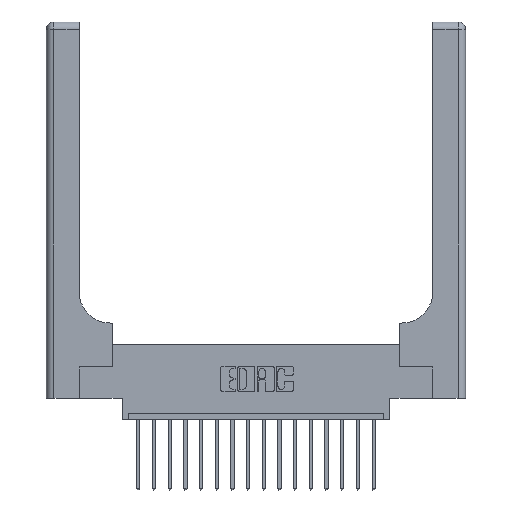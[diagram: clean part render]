
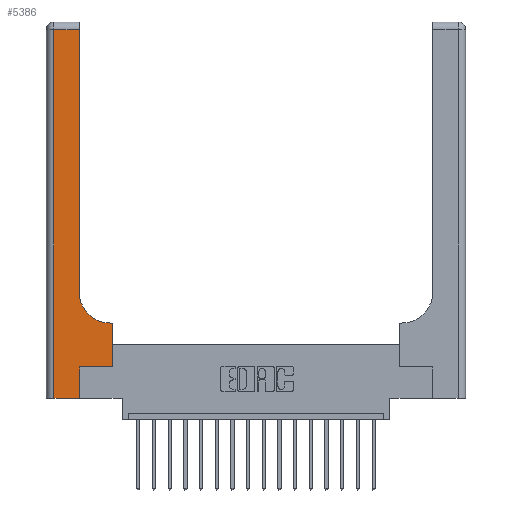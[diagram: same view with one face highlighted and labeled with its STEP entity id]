
A CAD part, top view. The second image highlights one B-rep face of the part: STEP entity #5386.
In plain terms, the highlighted planar face has unit normal (0, 0, 1).
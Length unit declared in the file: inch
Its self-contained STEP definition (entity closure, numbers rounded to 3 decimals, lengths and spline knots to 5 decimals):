
#7 = CARTESIAN_POINT ( 'NONE',  ( 0.51, 0.6, 0.37 ) ) ;
#153 = EDGE_CURVE ( 'NONE', #842, #13573, #8564, .T. ) ;
#242 = ORIENTED_EDGE ( 'NONE', *, *, #1094, .T. ) ;
#585 = EDGE_LOOP ( 'NONE', ( #3375, #5539, #4293, #13679, #2827, #242, #11772, #3308, #14104 ) ) ;
#842 = VERTEX_POINT ( 'NONE', #1672 ) ;
#946 = LINE ( 'NONE', #2567, #9885 ) ;
#1094 = EDGE_CURVE ( 'NONE', #7335, #13065, #18753, .T. ) ;
#1672 = CARTESIAN_POINT ( 'NONE',  ( 0.26, 2.94, 0.37 ) ) ;
#1750 = CARTESIAN_POINT ( 'NONE',  ( 0.528, 0.25, 0.37 ) ) ;
#2262 = LINE ( 'NONE', #8172, #13637 ) ;
#2374 = CARTESIAN_POINT ( 'NONE',  ( 0.265, 0., 0.37 ) ) ;
#2377 = DIRECTION ( 'NONE',  ( -1., 0., 0. ) ) ;
#2567 = CARTESIAN_POINT ( 'NONE',  ( 0.265, 0., 0.37 ) ) ;
#2792 = EDGE_CURVE ( 'NONE', #10053, #8790, #9748, .T. ) ;
#2827 = ORIENTED_EDGE ( 'NONE', *, *, #16114, .T. ) ;
#2954 = FACE_OUTER_BOUND ( 'NONE', #585, .T. ) ;
#3308 = ORIENTED_EDGE ( 'NONE', *, *, #16003, .T. ) ;
#3353 = VECTOR ( 'NONE', #17284, 39.37008 ) ;
#3375 = ORIENTED_EDGE ( 'NONE', *, *, #8252, .T. ) ;
#3729 = VERTEX_POINT ( 'NONE', #7 ) ;
#4293 = ORIENTED_EDGE ( 'NONE', *, *, #9003, .T. ) ;
#4323 = LINE ( 'NONE', #7350, #4621 ) ;
#4621 = VECTOR ( 'NONE', #8796, 39.37008 ) ;
#5386 = ADVANCED_FACE ( 'NONE', ( #2954 ), #8999, .F. ) ;
#5539 = ORIENTED_EDGE ( 'NONE', *, *, #153, .T. ) ;
#5937 = VECTOR ( 'NONE', #15556, 39.37008 ) ;
#6003 = CARTESIAN_POINT ( 'NONE',  ( 0.51, 0.85, 0.37 ) ) ;
#6724 = DIRECTION ( 'NONE',  ( -1., 0., 0. ) ) ;
#7335 = VERTEX_POINT ( 'NONE', #7520 ) ;
#7350 = CARTESIAN_POINT ( 'NONE',  ( 0.06, 3., 0.37 ) ) ;
#7520 = CARTESIAN_POINT ( 'NONE',  ( 0.265, 0.25, 0.37 ) ) ;
#7664 = CARTESIAN_POINT ( 'NONE',  ( 0.06, 2.94, 0.37 ) ) ;
#7982 = CARTESIAN_POINT ( 'NONE',  ( 0., 0., 0.37 ) ) ;
#8172 = CARTESIAN_POINT ( 'NONE',  ( 0.26, 3., 0.37 ) ) ;
#8252 = EDGE_CURVE ( 'NONE', #19178, #842, #2262, .T. ) ;
#8483 = AXIS2_PLACEMENT_3D ( 'NONE', #13485, #11516, #14742 ) ;
#8564 = LINE ( 'NONE', #17220, #13502 ) ;
#8790 = VERTEX_POINT ( 'NONE', #2374 ) ;
#8796 = DIRECTION ( 'NONE',  ( 0., -1., 0. ) ) ;
#8999 = PLANE ( 'NONE',  #8483 ) ;
#9003 = EDGE_CURVE ( 'NONE', #13573, #10053, #4323, .T. ) ;
#9748 = LINE ( 'NONE', #7982, #5937 ) ;
#9885 = VECTOR ( 'NONE', #11961, 39.37008 ) ;
#10053 = VERTEX_POINT ( 'NONE', #18555 ) ;
#11516 = DIRECTION ( 'NONE',  ( 0., 0., -1. ) ) ;
#11772 = ORIENTED_EDGE ( 'NONE', *, *, #12029, .T. ) ;
#11843 = DIRECTION ( 'NONE',  ( 0., 0., -1. ) ) ;
#11961 = DIRECTION ( 'NONE',  ( 0., 1., 0. ) ) ;
#12029 = EDGE_CURVE ( 'NONE', #13065, #13528, #12046, .T. ) ;
#12046 = LINE ( 'NONE', #1750, #16919 ) ;
#12207 = EDGE_CURVE ( 'NONE', #3729, #19178, #18794, .T. ) ;
#12336 = LINE ( 'NONE', #15693, #12689 ) ;
#12665 = DIRECTION ( 'NONE',  ( 0., 1., 0. ) ) ;
#12689 = VECTOR ( 'NONE', #2377, 39.37008 ) ;
#13065 = VERTEX_POINT ( 'NONE', #13197 ) ;
#13197 = CARTESIAN_POINT ( 'NONE',  ( 0.528, 0.25, 0.37 ) ) ;
#13229 = CARTESIAN_POINT ( 'NONE',  ( 0.528, 0.6, 0.37 ) ) ;
#13316 = CARTESIAN_POINT ( 'NONE',  ( 0.26, 0.85, 0.37 ) ) ;
#13485 = CARTESIAN_POINT ( 'NONE',  ( 0., 3., 0.37 ) ) ;
#13502 = VECTOR ( 'NONE', #6724, 39.37008 ) ;
#13528 = VERTEX_POINT ( 'NONE', #13229 ) ;
#13573 = VERTEX_POINT ( 'NONE', #7664 ) ;
#13637 = VECTOR ( 'NONE', #12665, 39.37008 ) ;
#13679 = ORIENTED_EDGE ( 'NONE', *, *, #2792, .T. ) ;
#14104 = ORIENTED_EDGE ( 'NONE', *, *, #12207, .T. ) ;
#14742 = DIRECTION ( 'NONE',  ( -1., 0., 0. ) ) ;
#15366 = AXIS2_PLACEMENT_3D ( 'NONE', #6003, #11843, #18085 ) ;
#15556 = DIRECTION ( 'NONE',  ( 1., 0., 0. ) ) ;
#15693 = CARTESIAN_POINT ( 'NONE',  ( 0.26, 0.6, 0.37 ) ) ;
#16003 = EDGE_CURVE ( 'NONE', #13528, #3729, #12336, .T. ) ;
#16114 = EDGE_CURVE ( 'NONE', #8790, #7335, #946, .T. ) ;
#16919 = VECTOR ( 'NONE', #18089, 39.37008 ) ;
#17220 = CARTESIAN_POINT ( 'NONE',  ( 0., 2.94, 0.37 ) ) ;
#17284 = DIRECTION ( 'NONE',  ( 1., 0., 0. ) ) ;
#18085 = DIRECTION ( 'NONE',  ( 1., 0., 0. ) ) ;
#18089 = DIRECTION ( 'NONE',  ( 0., 1., 0. ) ) ;
#18555 = CARTESIAN_POINT ( 'NONE',  ( 0.06, 0., 0.37 ) ) ;
#18560 = CARTESIAN_POINT ( 'NONE',  ( 0.265, 0.25, 0.37 ) ) ;
#18753 = LINE ( 'NONE', #18560, #3353 ) ;
#18794 = CIRCLE ( 'NONE', #15366, 0.25 ) ;
#19178 = VERTEX_POINT ( 'NONE', #13316 ) ;
